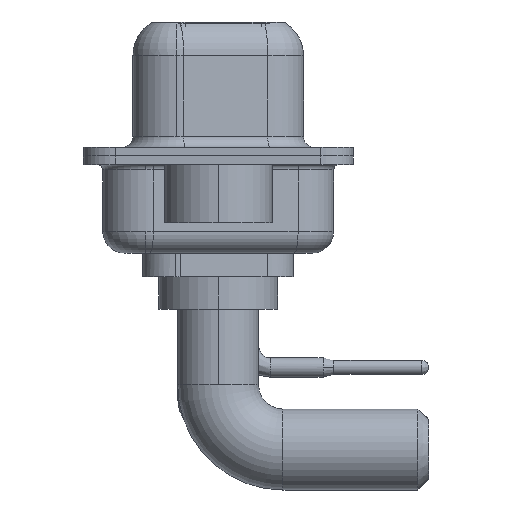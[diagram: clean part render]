
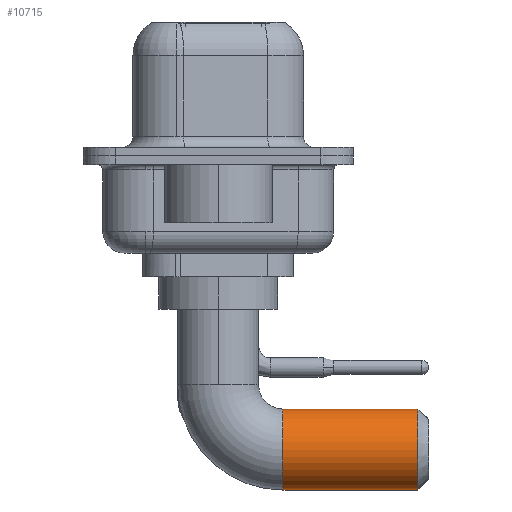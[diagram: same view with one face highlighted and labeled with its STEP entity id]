
A CAD part, left-side view. The second image highlights one B-rep face of the part: STEP entity #10715.
In plain terms, the highlighted cylindrical face has radius 1.875 mm (diameter 3.75 mm), a partial arc.
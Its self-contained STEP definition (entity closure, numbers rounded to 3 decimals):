
#575 = VERTEX_POINT ( 'NONE', #8976 ) ;
#767 = EDGE_CURVE ( 'NONE', #7638, #14883, #11447, .T. ) ;
#1011 = AXIS2_PLACEMENT_3D ( 'NONE', #7430, #12945, #6451 ) ;
#1980 = CARTESIAN_POINT ( 'NONE',  ( 0., -9.25, -6.5 ) ) ;
#2225 = ORIENTED_EDGE ( 'NONE', *, *, #7383, .T. ) ;
#2309 = ORIENTED_EDGE ( 'NONE', *, *, #767, .T. ) ;
#3221 = CARTESIAN_POINT ( 'NONE',  ( 0., -3., -8.375 ) ) ;
#3447 = CARTESIAN_POINT ( 'NONE',  ( 0., -3., -4.625 ) ) ;
#4665 = LINE ( 'NONE', #3447, #14828 ) ;
#4907 = ORIENTED_EDGE ( 'NONE', *, *, #12120, .T. ) ;
#5393 = DIRECTION ( 'NONE',  ( 0., -1., 0. ) ) ;
#6196 = CARTESIAN_POINT ( 'NONE',  ( 0., -3., -8.375 ) ) ;
#6451 = DIRECTION ( 'NONE',  ( 0., 0., -1. ) ) ;
#6671 = CARTESIAN_POINT ( 'NONE',  ( 0., -9.25, -8.375 ) ) ;
#6971 = EDGE_CURVE ( 'NONE', #7638, #575, #4665, .T. ) ;
#6985 = CARTESIAN_POINT ( 'NONE',  ( 0., -3., -4.625 ) ) ;
#7367 = ORIENTED_EDGE ( 'NONE', *, *, #6971, .F. ) ;
#7383 = EDGE_CURVE ( 'NONE', #14883, #13197, #10219, .T. ) ;
#7430 = CARTESIAN_POINT ( 'NONE',  ( 0., -3., -6.5 ) ) ;
#7607 = CYLINDRICAL_SURFACE ( 'NONE', #1011, 1.875 ) ;
#7638 = VERTEX_POINT ( 'NONE', #6985 ) ;
#8434 = EDGE_LOOP ( 'NONE', ( #7367, #2309, #2225, #4907 ) ) ;
#8659 = AXIS2_PLACEMENT_3D ( 'NONE', #15507, #5393, #14617 ) ;
#8976 = CARTESIAN_POINT ( 'NONE',  ( 0., -9.25, -4.625 ) ) ;
#10083 = DIRECTION ( 'NONE',  ( 0., 0., -1. ) ) ;
#10168 = DIRECTION ( 'NONE',  ( 0., 1., 0. ) ) ;
#10219 = LINE ( 'NONE', #6196, #15671 ) ;
#10715 = ADVANCED_FACE ( 'NONE', ( #14227 ), #7607, .T. ) ;
#11447 = CIRCLE ( 'NONE', #8659, 1.875 ) ;
#12120 = EDGE_CURVE ( 'NONE', #13197, #575, #16616, .T. ) ;
#12945 = DIRECTION ( 'NONE',  ( 0., -1., 0. ) ) ;
#13197 = VERTEX_POINT ( 'NONE', #6671 ) ;
#14077 = DIRECTION ( 'NONE',  ( 0., -1., 0. ) ) ;
#14227 = FACE_OUTER_BOUND ( 'NONE', #8434, .T. ) ;
#14617 = DIRECTION ( 'NONE',  ( -1., 0., 0. ) ) ;
#14828 = VECTOR ( 'NONE', #14077, 1000. ) ;
#14883 = VERTEX_POINT ( 'NONE', #3221 ) ;
#15273 = DIRECTION ( 'NONE',  ( 0., -1., 0. ) ) ;
#15507 = CARTESIAN_POINT ( 'NONE',  ( 0., -3., -6.5 ) ) ;
#15671 = VECTOR ( 'NONE', #15273, 1000. ) ;
#16058 = AXIS2_PLACEMENT_3D ( 'NONE', #1980, #10168, #10083 ) ;
#16616 = CIRCLE ( 'NONE', #16058, 1.875 ) ;
